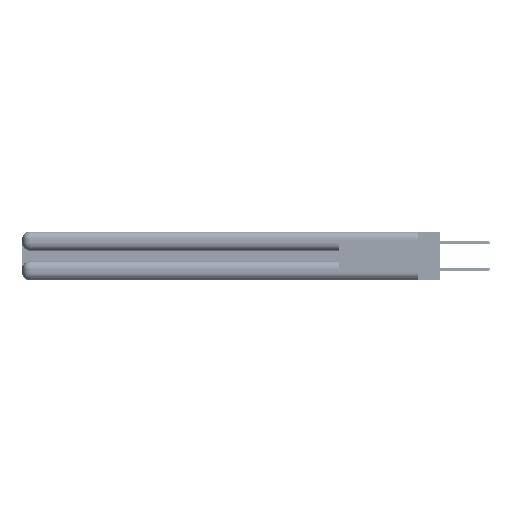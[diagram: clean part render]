
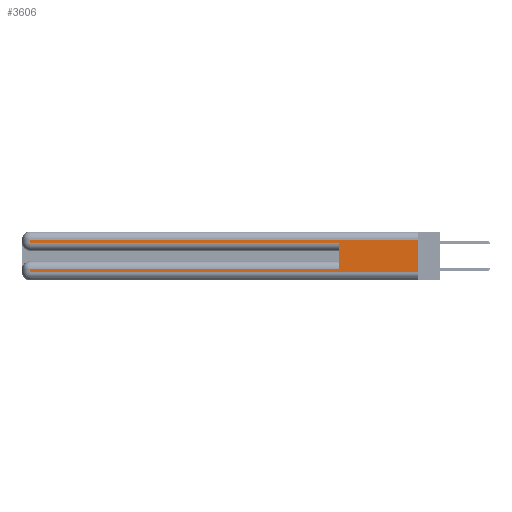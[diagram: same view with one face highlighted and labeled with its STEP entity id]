
A CAD part, left-side view. The second image highlights one B-rep face of the part: STEP entity #3606.
In plain terms, the highlighted planar face has unit normal (-1, 0, 0).
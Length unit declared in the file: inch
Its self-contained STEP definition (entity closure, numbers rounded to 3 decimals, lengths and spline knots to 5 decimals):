
#745 = CARTESIAN_POINT ( 'NONE',  ( 0., 2.94, 0.37 ) ) ;
#1084 = ORIENTED_EDGE ( 'NONE', *, *, #26943, .T. ) ;
#3606 = ADVANCED_FACE ( 'NONE', ( #5478 ), #29931, .F. ) ;
#3754 = CARTESIAN_POINT ( 'NONE',  ( 0., 0., 0.37 ) ) ;
#3832 = CARTESIAN_POINT ( 'NONE',  ( 0., 0., 0.31 ) ) ;
#3861 = CARTESIAN_POINT ( 'NONE',  ( 0., 0., 0.085 ) ) ;
#5151 = DIRECTION ( 'NONE',  ( 0., 0., -1. ) ) ;
#5478 = FACE_OUTER_BOUND ( 'NONE', #12647, .T. ) ;
#5510 = EDGE_CURVE ( 'NONE', #14861, #14514, #45624, .T. ) ;
#5677 = VECTOR ( 'NONE', #8215, 39.37008 ) ;
#6764 = AXIS2_PLACEMENT_3D ( 'NONE', #3754, #8137, #38688 ) ;
#7551 = CARTESIAN_POINT ( 'NONE',  ( 0., 2.94, 0.285 ) ) ;
#8137 = DIRECTION ( 'NONE',  ( 1., 0., 0. ) ) ;
#8215 = DIRECTION ( 'NONE',  ( 0., 1., 0. ) ) ;
#8243 = DIRECTION ( 'NONE',  ( 0., 1., 0. ) ) ;
#9079 = ORIENTED_EDGE ( 'NONE', *, *, #37792, .F. ) ;
#9168 = VERTEX_POINT ( 'NONE', #12348 ) ;
#9477 = VECTOR ( 'NONE', #11004, 39.37008 ) ;
#11004 = DIRECTION ( 'NONE',  ( 0., 0., -1. ) ) ;
#12348 = CARTESIAN_POINT ( 'NONE',  ( 0., 2.94, 0.085 ) ) ;
#12647 = EDGE_LOOP ( 'NONE', ( #9079, #29310, #22372, #43310, #30812, #22429, #15430, #1084 ) ) ;
#13039 = CARTESIAN_POINT ( 'NONE',  ( 0., 0., 0.06 ) ) ;
#14514 = VERTEX_POINT ( 'NONE', #34725 ) ;
#14660 = VECTOR ( 'NONE', #19215, 39.37008 ) ;
#14780 = EDGE_CURVE ( 'NONE', #39414, #14514, #20099, .T. ) ;
#14861 = VERTEX_POINT ( 'NONE', #38140 ) ;
#15430 = ORIENTED_EDGE ( 'NONE', *, *, #31682, .T. ) ;
#17413 = EDGE_CURVE ( 'NONE', #27789, #25710, #40506, .T. ) ;
#17466 = VERTEX_POINT ( 'NONE', #13039 ) ;
#19215 = DIRECTION ( 'NONE',  ( 0., -1., 0. ) ) ;
#20099 = LINE ( 'NONE', #41749, #41872 ) ;
#21381 = EDGE_CURVE ( 'NONE', #25710, #39414, #52973, .T. ) ;
#22372 = ORIENTED_EDGE ( 'NONE', *, *, #21381, .T. ) ;
#22429 = ORIENTED_EDGE ( 'NONE', *, *, #40189, .T. ) ;
#22494 = LINE ( 'NONE', #37107, #9477 ) ;
#24377 = CARTESIAN_POINT ( 'NONE',  ( 0., 2.94, 0.37 ) ) ;
#25710 = VERTEX_POINT ( 'NONE', #54702 ) ;
#26300 = VECTOR ( 'NONE', #5151, 39.37008 ) ;
#26943 = EDGE_CURVE ( 'NONE', #40175, #17466, #49377, .T. ) ;
#27789 = VERTEX_POINT ( 'NONE', #38917 ) ;
#29310 = ORIENTED_EDGE ( 'NONE', *, *, #17413, .T. ) ;
#29931 = PLANE ( 'NONE',  #6764 ) ;
#30812 = ORIENTED_EDGE ( 'NONE', *, *, #5510, .F. ) ;
#31682 = EDGE_CURVE ( 'NONE', #9168, #40175, #49427, .T. ) ;
#33103 = DIRECTION ( 'NONE',  ( 0., 0., -1. ) ) ;
#34034 = VECTOR ( 'NONE', #47807, 39.37008 ) ;
#34725 = CARTESIAN_POINT ( 'NONE',  ( 0., 0.6, 0.285 ) ) ;
#35800 = VECTOR ( 'NONE', #8243, 39.37008 ) ;
#37107 = CARTESIAN_POINT ( 'NONE',  ( 0., 0., 0.37 ) ) ;
#37183 = LINE ( 'NONE', #3861, #35800 ) ;
#37792 = EDGE_CURVE ( 'NONE', #27789, #17466, #22494, .T. ) ;
#38140 = CARTESIAN_POINT ( 'NONE',  ( 0., 0.6, 0.085 ) ) ;
#38688 = DIRECTION ( 'NONE',  ( 0., 0., -1. ) ) ;
#38917 = CARTESIAN_POINT ( 'NONE',  ( 0., 0., 0.31 ) ) ;
#39414 = VERTEX_POINT ( 'NONE', #7551 ) ;
#40175 = VERTEX_POINT ( 'NONE', #56090 ) ;
#40189 = EDGE_CURVE ( 'NONE', #14861, #9168, #37183, .T. ) ;
#40506 = LINE ( 'NONE', #3832, #5677 ) ;
#41749 = CARTESIAN_POINT ( 'NONE',  ( 0., 0., 0.285 ) ) ;
#41872 = VECTOR ( 'NONE', #46125, 39.37008 ) ;
#43310 = ORIENTED_EDGE ( 'NONE', *, *, #14780, .T. ) ;
#45624 = LINE ( 'NONE', #56367, #34034 ) ;
#46125 = DIRECTION ( 'NONE',  ( 0., -1., 0. ) ) ;
#47807 = DIRECTION ( 'NONE',  ( 0., 0., 1. ) ) ;
#49377 = LINE ( 'NONE', #49637, #14660 ) ;
#49427 = LINE ( 'NONE', #745, #26300 ) ;
#49637 = CARTESIAN_POINT ( 'NONE',  ( 0., 0., 0.06 ) ) ;
#51591 = VECTOR ( 'NONE', #33103, 39.37008 ) ;
#52973 = LINE ( 'NONE', #24377, #51591 ) ;
#54702 = CARTESIAN_POINT ( 'NONE',  ( 0., 2.94, 0.31 ) ) ;
#56090 = CARTESIAN_POINT ( 'NONE',  ( 0., 2.94, 0.06 ) ) ;
#56367 = CARTESIAN_POINT ( 'NONE',  ( 0., 0.6, 0.145 ) ) ;
